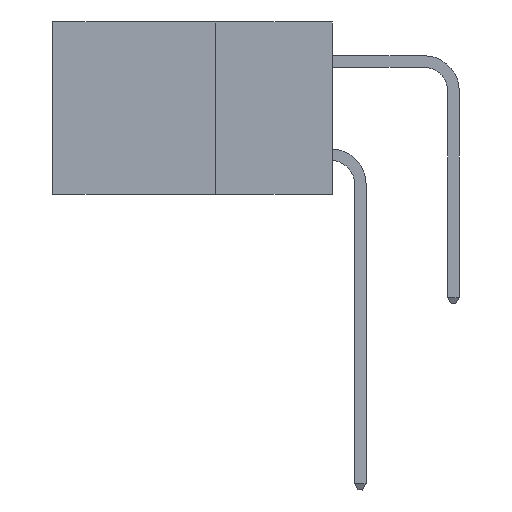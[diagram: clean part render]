
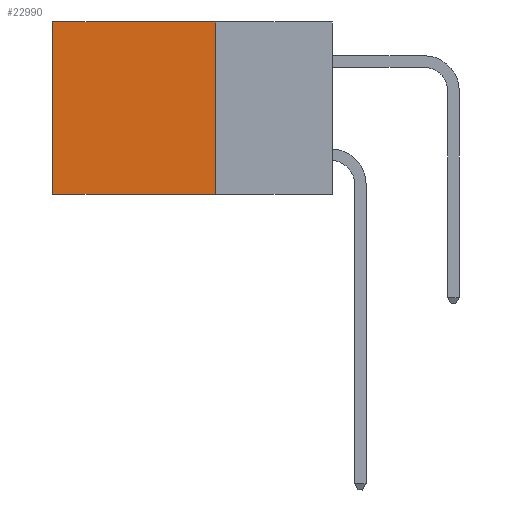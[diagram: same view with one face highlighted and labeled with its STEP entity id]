
A CAD part, left-side view. The second image highlights one B-rep face of the part: STEP entity #22990.
In plain terms, the highlighted planar face has unit normal (-1, 0, 0).
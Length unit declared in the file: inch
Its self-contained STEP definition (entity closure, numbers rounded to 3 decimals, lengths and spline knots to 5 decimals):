
#527 = VERTEX_POINT ( 'NONE', #17635 ) ;
#573 = EDGE_LOOP ( 'NONE', ( #19709, #2678, #15194, #21579 ) ) ;
#940 = FACE_OUTER_BOUND ( 'NONE', #573, .T. ) ;
#1137 = EDGE_CURVE ( 'NONE', #21726, #527, #8604, .T. ) ;
#2585 = DIRECTION ( 'NONE',  ( 1., 0., 0. ) ) ;
#2678 = ORIENTED_EDGE ( 'NONE', *, *, #5165, .F. ) ;
#2840 = CARTESIAN_POINT ( 'NONE',  ( 0.2615, 0.25, -0.37 ) ) ;
#2957 = CARTESIAN_POINT ( 'NONE',  ( 0.2615, 0.25, -0.37 ) ) ;
#3111 = VECTOR ( 'NONE', #6549, 39.37008 ) ;
#3320 = LINE ( 'NONE', #6551, #6179 ) ;
#4071 = CARTESIAN_POINT ( 'NONE',  ( 0.2615, 0.6, 0. ) ) ;
#4886 = DIRECTION ( 'NONE',  ( 0., 0., -1. ) ) ;
#5119 = CARTESIAN_POINT ( 'NONE',  ( 0.2615, 0.6, -0.37 ) ) ;
#5165 = EDGE_CURVE ( 'NONE', #527, #22443, #3320, .T. ) ;
#5251 = EDGE_CURVE ( 'NONE', #15331, #22443, #6424, .T. ) ;
#6065 = LINE ( 'NONE', #16205, #17083 ) ;
#6179 = VECTOR ( 'NONE', #22776, 39.37008 ) ;
#6424 = LINE ( 'NONE', #5119, #18888 ) ;
#6549 = DIRECTION ( 'NONE',  ( 0., 0., -1. ) ) ;
#6551 = CARTESIAN_POINT ( 'NONE',  ( 0.2615, 0.25, -0.37 ) ) ;
#8604 = LINE ( 'NONE', #2840, #3111 ) ;
#10265 = PLANE ( 'NONE',  #24779 ) ;
#12702 = CARTESIAN_POINT ( 'NONE',  ( 0.2615, 0.25, 0. ) ) ;
#13812 = CARTESIAN_POINT ( 'NONE',  ( 0.2615, 0.6, -0.37 ) ) ;
#15194 = ORIENTED_EDGE ( 'NONE', *, *, #1137, .F. ) ;
#15331 = VERTEX_POINT ( 'NONE', #4071 ) ;
#15948 = DIRECTION ( 'NONE',  ( 0., 1., 0. ) ) ;
#16205 = CARTESIAN_POINT ( 'NONE',  ( 0.2615, 0.25, 0. ) ) ;
#17083 = VECTOR ( 'NONE', #15948, 39.37008 ) ;
#17635 = CARTESIAN_POINT ( 'NONE',  ( 0.2615, 0.25, -0.37 ) ) ;
#18888 = VECTOR ( 'NONE', #24817, 39.37008 ) ;
#19709 = ORIENTED_EDGE ( 'NONE', *, *, #5251, .T. ) ;
#21579 = ORIENTED_EDGE ( 'NONE', *, *, #24494, .T. ) ;
#21726 = VERTEX_POINT ( 'NONE', #12702 ) ;
#22443 = VERTEX_POINT ( 'NONE', #13812 ) ;
#22776 = DIRECTION ( 'NONE',  ( 0., 1., 0. ) ) ;
#22990 = ADVANCED_FACE ( 'NONE', ( #940 ), #10265, .F. ) ;
#24494 = EDGE_CURVE ( 'NONE', #21726, #15331, #6065, .T. ) ;
#24779 = AXIS2_PLACEMENT_3D ( 'NONE', #2957, #2585, #4886 ) ;
#24817 = DIRECTION ( 'NONE',  ( 0., 0., -1. ) ) ;
